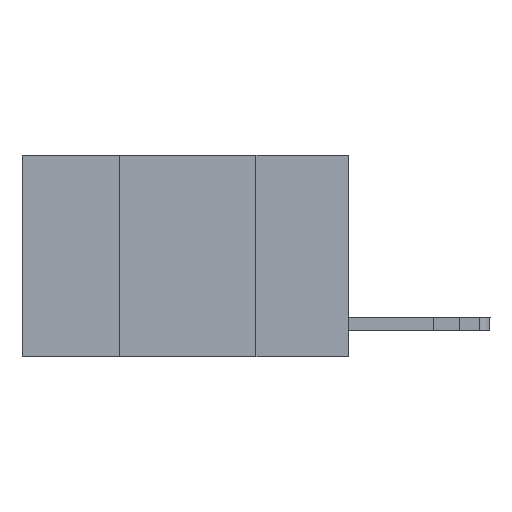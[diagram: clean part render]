
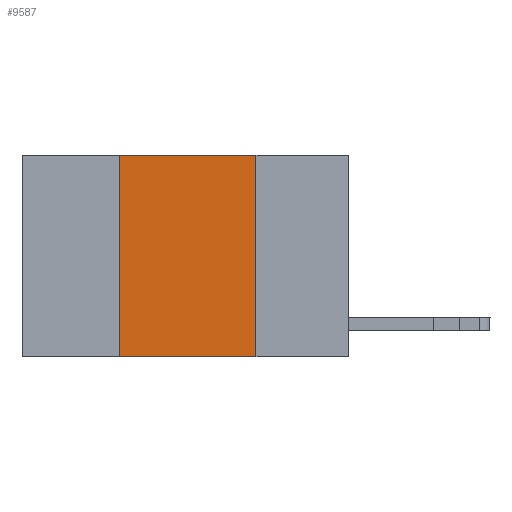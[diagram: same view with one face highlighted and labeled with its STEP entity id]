
A CAD part, left-side view. The second image highlights one B-rep face of the part: STEP entity #9587.
In plain terms, the highlighted planar face has unit normal (-1, 0, 0).
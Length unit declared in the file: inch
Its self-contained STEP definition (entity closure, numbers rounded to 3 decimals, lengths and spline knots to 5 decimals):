
#379 = VECTOR ( 'NONE', #12456, 39.37008 ) ;
#666 = VECTOR ( 'NONE', #12211, 39.37008 ) ;
#748 = VECTOR ( 'NONE', #6695, 39.37008 ) ;
#823 = VERTEX_POINT ( 'NONE', #2365 ) ;
#1431 = EDGE_LOOP ( 'NONE', ( #4878, #2219, #8596, #3233 ) ) ;
#1892 = VERTEX_POINT ( 'NONE', #8652 ) ;
#1909 = LINE ( 'NONE', #5332, #666 ) ;
#2219 = ORIENTED_EDGE ( 'NONE', *, *, #12283, .F. ) ;
#2365 = CARTESIAN_POINT ( 'NONE',  ( 0., 0.42, 0. ) ) ;
#3219 = CARTESIAN_POINT ( 'NONE',  ( 0., 0.6, 0. ) ) ;
#3233 = ORIENTED_EDGE ( 'NONE', *, *, #9917, .T. ) ;
#3602 = EDGE_CURVE ( 'NONE', #1892, #8620, #1909, .T. ) ;
#4150 = CARTESIAN_POINT ( 'NONE',  ( 0., 0.42, 0. ) ) ;
#4330 = CARTESIAN_POINT ( 'NONE',  ( 0., 0.6, -0.37 ) ) ;
#4878 = ORIENTED_EDGE ( 'NONE', *, *, #3602, .F. ) ;
#5262 = FACE_OUTER_BOUND ( 'NONE', #1431, .T. ) ;
#5332 = CARTESIAN_POINT ( 'NONE',  ( 0., 0.17, 0. ) ) ;
#5467 = DIRECTION ( 'NONE',  ( 1., 0., 0. ) ) ;
#6047 = CARTESIAN_POINT ( 'NONE',  ( 0., 0.17, -0.37 ) ) ;
#6365 = PLANE ( 'NONE',  #10654 ) ;
#6695 = DIRECTION ( 'NONE',  ( 0., -1., 0. ) ) ;
#7441 = VECTOR ( 'NONE', #11922, 39.37008 ) ;
#7611 = EDGE_CURVE ( 'NONE', #13769, #823, #14347, .T. ) ;
#7926 = LINE ( 'NONE', #4330, #748 ) ;
#8596 = ORIENTED_EDGE ( 'NONE', *, *, #7611, .F. ) ;
#8620 = VERTEX_POINT ( 'NONE', #6047 ) ;
#8652 = CARTESIAN_POINT ( 'NONE',  ( 0., 0.17, 0. ) ) ;
#9107 = CARTESIAN_POINT ( 'NONE',  ( 0., 0.42, -0.37 ) ) ;
#9587 = ADVANCED_FACE ( 'NONE', ( #5262 ), #6365, .F. ) ;
#9917 = EDGE_CURVE ( 'NONE', #13769, #8620, #7926, .T. ) ;
#10654 = AXIS2_PLACEMENT_3D ( 'NONE', #12216, #5467, #14522 ) ;
#11922 = DIRECTION ( 'NONE',  ( 0., 0., 1. ) ) ;
#12211 = DIRECTION ( 'NONE',  ( 0., 0., -1. ) ) ;
#12216 = CARTESIAN_POINT ( 'NONE',  ( 0., 0.6, 0. ) ) ;
#12283 = EDGE_CURVE ( 'NONE', #823, #1892, #12302, .T. ) ;
#12302 = LINE ( 'NONE', #3219, #379 ) ;
#12456 = DIRECTION ( 'NONE',  ( 0., -1., 0. ) ) ;
#13769 = VERTEX_POINT ( 'NONE', #9107 ) ;
#14347 = LINE ( 'NONE', #4150, #7441 ) ;
#14522 = DIRECTION ( 'NONE',  ( 0., 0., -1. ) ) ;
